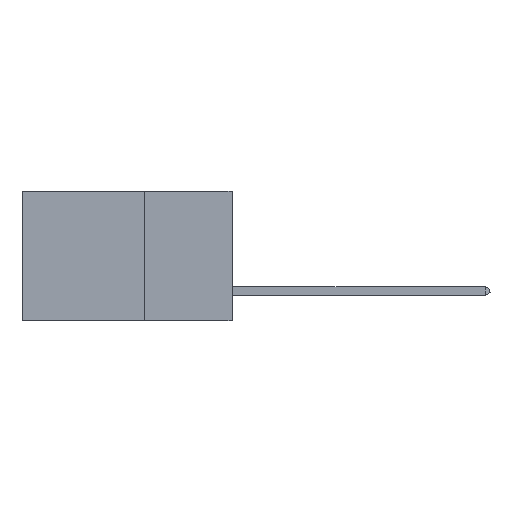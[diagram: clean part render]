
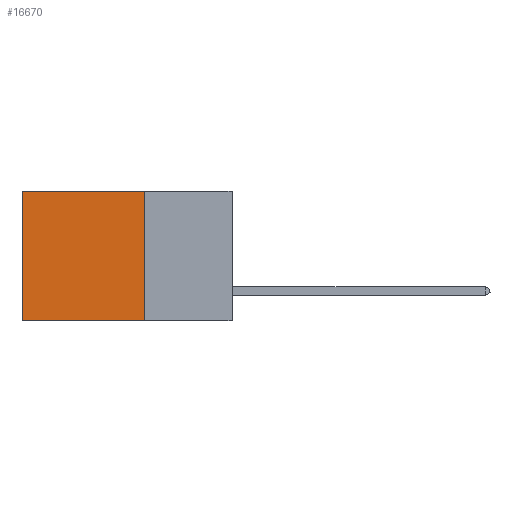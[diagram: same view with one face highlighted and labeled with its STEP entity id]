
A CAD part, left-side view. The second image highlights one B-rep face of the part: STEP entity #16670.
In plain terms, the highlighted planar face has unit normal (-1, 0, 0).
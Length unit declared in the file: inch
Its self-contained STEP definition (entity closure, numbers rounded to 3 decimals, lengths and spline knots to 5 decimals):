
#265 = LINE ( 'NONE', #12568, #16839 ) ;
#1049 = VERTEX_POINT ( 'NONE', #8896 ) ;
#1119 = EDGE_CURVE ( 'NONE', #5752, #1049, #265, .T. ) ;
#1512 = EDGE_LOOP ( 'NONE', ( #13039, #2323, #5942, #3790 ) ) ;
#1842 = EDGE_CURVE ( 'NONE', #15727, #1049, #7267, .T. ) ;
#2323 = ORIENTED_EDGE ( 'NONE', *, *, #1842, .F. ) ;
#2718 = VECTOR ( 'NONE', #4112, 39.37008 ) ;
#3117 = DIRECTION ( 'NONE',  ( 0., 0., -1. ) ) ;
#3786 = VERTEX_POINT ( 'NONE', #14693 ) ;
#3790 = ORIENTED_EDGE ( 'NONE', *, *, #12087, .T. ) ;
#4112 = DIRECTION ( 'NONE',  ( 0., 1., 0. ) ) ;
#4610 = CARTESIAN_POINT ( 'NONE',  ( 0.2875, 0.6, 0. ) ) ;
#5468 = CARTESIAN_POINT ( 'NONE',  ( 0.2875, 0.25, 0. ) ) ;
#5752 = VERTEX_POINT ( 'NONE', #4610 ) ;
#5874 = DIRECTION ( 'NONE',  ( 0., 1., 0. ) ) ;
#5942 = ORIENTED_EDGE ( 'NONE', *, *, #13732, .F. ) ;
#6963 = PLANE ( 'NONE',  #12468 ) ;
#7267 = LINE ( 'NONE', #12684, #13761 ) ;
#8356 = DIRECTION ( 'NONE',  ( 1., 0., 0. ) ) ;
#8896 = CARTESIAN_POINT ( 'NONE',  ( 0.2875, 0.6, -0.37 ) ) ;
#9739 = DIRECTION ( 'NONE',  ( 0., 0., -1. ) ) ;
#10805 = LINE ( 'NONE', #5468, #17724 ) ;
#12087 = EDGE_CURVE ( 'NONE', #3786, #5752, #12588, .T. ) ;
#12123 = FACE_OUTER_BOUND ( 'NONE', #1512, .T. ) ;
#12352 = CARTESIAN_POINT ( 'NONE',  ( 0.2875, 0.25, 0. ) ) ;
#12468 = AXIS2_PLACEMENT_3D ( 'NONE', #16646, #8356, #9739 ) ;
#12568 = CARTESIAN_POINT ( 'NONE',  ( 0.2875, 0.6, 0. ) ) ;
#12588 = LINE ( 'NONE', #12352, #2718 ) ;
#12684 = CARTESIAN_POINT ( 'NONE',  ( 0.2875, 0.25, -0.37 ) ) ;
#13039 = ORIENTED_EDGE ( 'NONE', *, *, #1119, .T. ) ;
#13732 = EDGE_CURVE ( 'NONE', #3786, #15727, #10805, .T. ) ;
#13761 = VECTOR ( 'NONE', #5874, 39.37008 ) ;
#14169 = CARTESIAN_POINT ( 'NONE',  ( 0.2875, 0.25, -0.37 ) ) ;
#14693 = CARTESIAN_POINT ( 'NONE',  ( 0.2875, 0.25, 0. ) ) ;
#15727 = VERTEX_POINT ( 'NONE', #14169 ) ;
#16532 = DIRECTION ( 'NONE',  ( 0., 0., -1. ) ) ;
#16646 = CARTESIAN_POINT ( 'NONE',  ( 0.2875, 0.25, 0. ) ) ;
#16670 = ADVANCED_FACE ( 'NONE', ( #12123 ), #6963, .F. ) ;
#16839 = VECTOR ( 'NONE', #3117, 39.37008 ) ;
#17724 = VECTOR ( 'NONE', #16532, 39.37008 ) ;
